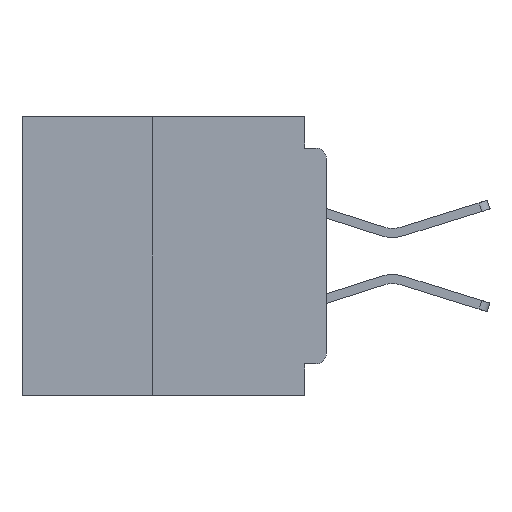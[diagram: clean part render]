
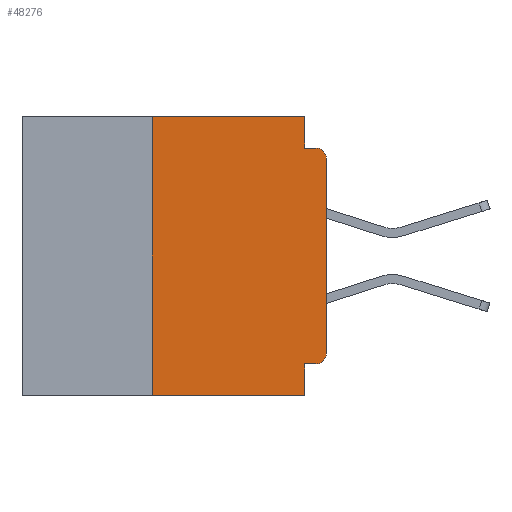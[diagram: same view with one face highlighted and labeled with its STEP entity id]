
A CAD part, left-side view. The second image highlights one B-rep face of the part: STEP entity #48276.
In plain terms, the highlighted planar face has unit normal (-1, 0, 0).
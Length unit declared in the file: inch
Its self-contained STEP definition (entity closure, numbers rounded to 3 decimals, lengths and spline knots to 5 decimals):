
#129 = EDGE_CURVE ( 'NONE', #4989, #7237, #3267, .T. ) ;
#139 = LINE ( 'NONE', #38123, #38023 ) ;
#812 = EDGE_CURVE ( 'NONE', #11053, #32435, #16365, .T. ) ;
#1068 = EDGE_LOOP ( 'NONE', ( #11328, #8710, #7946, #45069, #43194, #37602, #25088, #33185, #17873, #35354 ) ) ;
#1246 = DIRECTION ( 'NONE',  ( 1., 0., 0. ) ) ;
#1296 = VECTOR ( 'NONE', #9013, 39.37008 ) ;
#1952 = DIRECTION ( 'NONE',  ( 0., 0., -1. ) ) ;
#2540 = VERTEX_POINT ( 'NONE', #46787 ) ;
#3267 = LINE ( 'NONE', #10236, #42260 ) ;
#4758 = LINE ( 'NONE', #6670, #31303 ) ;
#4989 = VERTEX_POINT ( 'NONE', #12777 ) ;
#5021 = VECTOR ( 'NONE', #12874, 39.37008 ) ;
#5366 = CARTESIAN_POINT ( 'NONE',  ( 0., 0.031, 0. ) ) ;
#5668 = VECTOR ( 'NONE', #13766, 39.37008 ) ;
#6670 = CARTESIAN_POINT ( 'NONE',  ( 0., 0.25, -0.4 ) ) ;
#7237 = VERTEX_POINT ( 'NONE', #46919 ) ;
#7257 = DIRECTION ( 'NONE',  ( -1., 0., 0. ) ) ;
#7644 = CARTESIAN_POINT ( 'NONE',  ( 0., 0.031, 0. ) ) ;
#7946 = ORIENTED_EDGE ( 'NONE', *, *, #812, .F. ) ;
#8018 = VERTEX_POINT ( 'NONE', #25419 ) ;
#8710 = ORIENTED_EDGE ( 'NONE', *, *, #10059, .T. ) ;
#9013 = DIRECTION ( 'NONE',  ( 0., 0., 1. ) ) ;
#9364 = DIRECTION ( 'NONE',  ( 0., 1., 0. ) ) ;
#10059 = EDGE_CURVE ( 'NONE', #2540, #32435, #18378, .T. ) ;
#10236 = CARTESIAN_POINT ( 'NONE',  ( 0., 0., -0.355 ) ) ;
#10546 = DIRECTION ( 'NONE',  ( 0., 0., 1. ) ) ;
#11053 = VERTEX_POINT ( 'NONE', #31497 ) ;
#11328 = ORIENTED_EDGE ( 'NONE', *, *, #29651, .T. ) ;
#11912 = DIRECTION ( 'NONE',  ( 0., 0., -1. ) ) ;
#12648 = EDGE_CURVE ( 'NONE', #17338, #11053, #47715, .T. ) ;
#12716 = EDGE_CURVE ( 'NONE', #4989, #8018, #34802, .T. ) ;
#12742 = CARTESIAN_POINT ( 'NONE',  ( 0., 0., -0.045 ) ) ;
#12777 = CARTESIAN_POINT ( 'NONE',  ( 0., 0.015, -0.355 ) ) ;
#12835 = CARTESIAN_POINT ( 'NONE',  ( 0., 0., 0. ) ) ;
#12874 = DIRECTION ( 'NONE',  ( 0., -1., 0. ) ) ;
#13766 = DIRECTION ( 'NONE',  ( 0., -1., 0. ) ) ;
#14342 = CARTESIAN_POINT ( 'NONE',  ( 0., 0.437, -0.4 ) ) ;
#16188 = EDGE_CURVE ( 'NONE', #7237, #33314, #139, .T. ) ;
#16365 = LINE ( 'NONE', #12742, #5021 ) ;
#17338 = VERTEX_POINT ( 'NONE', #7644 ) ;
#17791 = CARTESIAN_POINT ( 'NONE',  ( 0., 0.25, 0. ) ) ;
#17873 = ORIENTED_EDGE ( 'NONE', *, *, #129, .F. ) ;
#18378 = CIRCLE ( 'NONE', #28414, 0.015 ) ;
#18494 = VECTOR ( 'NONE', #31732, 39.37008 ) ;
#22262 = CARTESIAN_POINT ( 'NONE',  ( 0., 0.031, -0.4 ) ) ;
#23242 = EDGE_CURVE ( 'NONE', #27877, #33314, #34400, .T. ) ;
#24062 = CARTESIAN_POINT ( 'NONE',  ( 0., 0.437, 0. ) ) ;
#24532 = VECTOR ( 'NONE', #40410, 39.37008 ) ;
#24745 = DIRECTION ( 'NONE',  ( -1., 0., 0. ) ) ;
#25088 = ORIENTED_EDGE ( 'NONE', *, *, #23242, .T. ) ;
#25419 = CARTESIAN_POINT ( 'NONE',  ( 0., 0., -0.34 ) ) ;
#27807 = DIRECTION ( 'NONE',  ( 0., 0., -1. ) ) ;
#27877 = VERTEX_POINT ( 'NONE', #32939 ) ;
#28414 = AXIS2_PLACEMENT_3D ( 'NONE', #29808, #7257, #33528 ) ;
#28494 = EDGE_CURVE ( 'NONE', #32411, #17338, #46895, .T. ) ;
#29651 = EDGE_CURVE ( 'NONE', #8018, #2540, #41535, .T. ) ;
#29808 = CARTESIAN_POINT ( 'NONE',  ( 0., 0.015, -0.06 ) ) ;
#31303 = VECTOR ( 'NONE', #10546, 39.37008 ) ;
#31497 = CARTESIAN_POINT ( 'NONE',  ( 0., 0.031, -0.045 ) ) ;
#31732 = DIRECTION ( 'NONE',  ( 0., 0., -1. ) ) ;
#32411 = VERTEX_POINT ( 'NONE', #17791 ) ;
#32435 = VERTEX_POINT ( 'NONE', #36724 ) ;
#32939 = CARTESIAN_POINT ( 'NONE',  ( 0., 0.25, -0.4 ) ) ;
#33185 = ORIENTED_EDGE ( 'NONE', *, *, #16188, .F. ) ;
#33314 = VERTEX_POINT ( 'NONE', #22262 ) ;
#33528 = DIRECTION ( 'NONE',  ( 0., 0., -1. ) ) ;
#34400 = LINE ( 'NONE', #14342, #24532 ) ;
#34802 = CIRCLE ( 'NONE', #36625, 0.015 ) ;
#35354 = ORIENTED_EDGE ( 'NONE', *, *, #12716, .T. ) ;
#35414 = FACE_OUTER_BOUND ( 'NONE', #1068, .T. ) ;
#36625 = AXIS2_PLACEMENT_3D ( 'NONE', #47166, #24745, #1952 ) ;
#36724 = CARTESIAN_POINT ( 'NONE',  ( 0., 0.015, -0.045 ) ) ;
#37602 = ORIENTED_EDGE ( 'NONE', *, *, #48529, .F. ) ;
#38023 = VECTOR ( 'NONE', #11912, 39.37008 ) ;
#38123 = CARTESIAN_POINT ( 'NONE',  ( 0., 0.031, -0.4 ) ) ;
#40002 = CARTESIAN_POINT ( 'NONE',  ( 0., 0.437, 0. ) ) ;
#40410 = DIRECTION ( 'NONE',  ( 0., -1., 0. ) ) ;
#41535 = LINE ( 'NONE', #12835, #1296 ) ;
#42260 = VECTOR ( 'NONE', #9364, 39.37008 ) ;
#43194 = ORIENTED_EDGE ( 'NONE', *, *, #28494, .F. ) ;
#44865 = AXIS2_PLACEMENT_3D ( 'NONE', #24062, #1246, #27807 ) ;
#45069 = ORIENTED_EDGE ( 'NONE', *, *, #12648, .F. ) ;
#46483 = PLANE ( 'NONE',  #44865 ) ;
#46787 = CARTESIAN_POINT ( 'NONE',  ( 0., 0., -0.06 ) ) ;
#46895 = LINE ( 'NONE', #40002, #5668 ) ;
#46919 = CARTESIAN_POINT ( 'NONE',  ( 0., 0.031, -0.355 ) ) ;
#47166 = CARTESIAN_POINT ( 'NONE',  ( 0., 0.015, -0.34 ) ) ;
#47715 = LINE ( 'NONE', #5366, #18494 ) ;
#48276 = ADVANCED_FACE ( 'NONE', ( #35414 ), #46483, .F. ) ;
#48529 = EDGE_CURVE ( 'NONE', #27877, #32411, #4758, .T. ) ;
